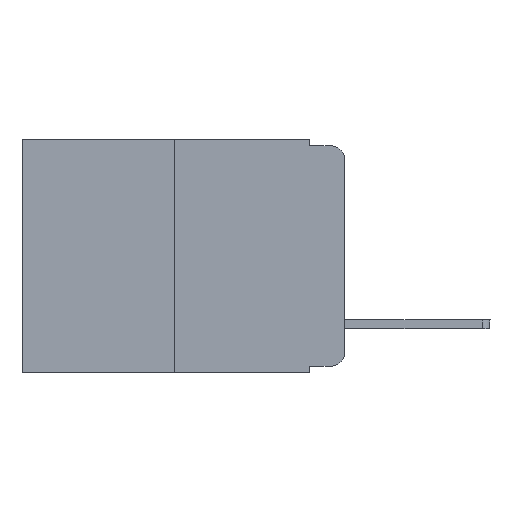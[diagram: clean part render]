
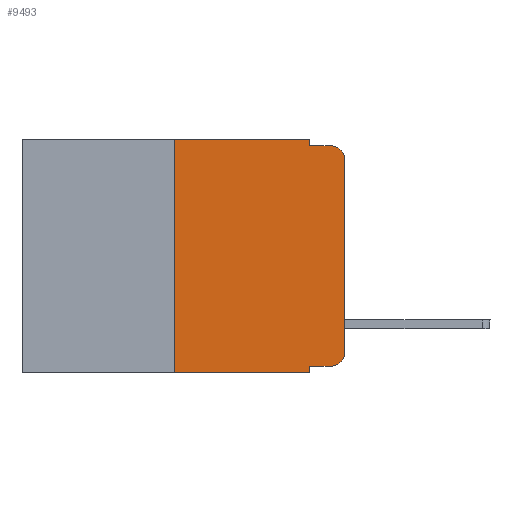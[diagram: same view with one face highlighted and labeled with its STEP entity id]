
A CAD part, left-side view. The second image highlights one B-rep face of the part: STEP entity #9493.
In plain terms, the highlighted planar face has unit normal (-1, 0, 0).
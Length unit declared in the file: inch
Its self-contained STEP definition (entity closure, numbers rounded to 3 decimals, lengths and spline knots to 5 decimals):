
#215 = VECTOR ( 'NONE', #10803, 39.37008 ) ;
#289 = DIRECTION ( 'NONE',  ( 0., 0., 1. ) ) ;
#607 = EDGE_CURVE ( 'NONE', #8277, #5988, #11055, .T. ) ;
#643 = VERTEX_POINT ( 'NONE', #4210 ) ;
#698 = DIRECTION ( 'NONE',  ( 0., 0., -1. ) ) ;
#714 = LINE ( 'NONE', #9930, #3446 ) ;
#875 = DIRECTION ( 'NONE',  ( 1., 0., 0. ) ) ;
#1143 = VECTOR ( 'NONE', #3246, 39.37008 ) ;
#1357 = VERTEX_POINT ( 'NONE', #4005 ) ;
#1798 = ORIENTED_EDGE ( 'NONE', *, *, #607, .F. ) ;
#1890 = EDGE_CURVE ( 'NONE', #4955, #5988, #4414, .T. ) ;
#2115 = AXIS2_PLACEMENT_3D ( 'NONE', #11380, #875, #698 ) ;
#2176 = VECTOR ( 'NONE', #10593, 39.37008 ) ;
#2335 = CARTESIAN_POINT ( 'NONE',  ( 0., 0.051, -0.01 ) ) ;
#2365 = ORIENTED_EDGE ( 'NONE', *, *, #10580, .F. ) ;
#2372 = CARTESIAN_POINT ( 'NONE',  ( 0., 0.25, 0. ) ) ;
#2379 = EDGE_CURVE ( 'NONE', #1357, #10682, #8162, .T. ) ;
#2500 = VERTEX_POINT ( 'NONE', #10598 ) ;
#2794 = LINE ( 'NONE', #2843, #2176 ) ;
#2843 = CARTESIAN_POINT ( 'NONE',  ( 0., 0.473, 0. ) ) ;
#2979 = VERTEX_POINT ( 'NONE', #6728 ) ;
#3246 = DIRECTION ( 'NONE',  ( 0., 0., 1. ) ) ;
#3319 = EDGE_CURVE ( 'NONE', #10682, #2979, #7691, .T. ) ;
#3352 = VECTOR ( 'NONE', #9895, 39.37008 ) ;
#3446 = VECTOR ( 'NONE', #289, 39.37008 ) ;
#3928 = DIRECTION ( 'NONE',  ( 0., -1., 0. ) ) ;
#3960 = CIRCLE ( 'NONE', #7475, 0.02 ) ;
#4005 = CARTESIAN_POINT ( 'NONE',  ( 0., 0.051, 0. ) ) ;
#4210 = CARTESIAN_POINT ( 'NONE',  ( 0., 0.02, -0.333 ) ) ;
#4268 = ORIENTED_EDGE ( 'NONE', *, *, #1890, .T. ) ;
#4309 = DIRECTION ( 'NONE',  ( 0., -1., 0. ) ) ;
#4394 = CARTESIAN_POINT ( 'NONE',  ( 0., 0.02, -0.313 ) ) ;
#4414 = LINE ( 'NONE', #8666, #8028 ) ;
#4492 = DIRECTION ( 'NONE',  ( 0., 0., -1. ) ) ;
#4650 = EDGE_CURVE ( 'NONE', #4955, #5913, #9793, .T. ) ;
#4844 = CARTESIAN_POINT ( 'NONE',  ( 0., 0., -0.03 ) ) ;
#4903 = FACE_OUTER_BOUND ( 'NONE', #11170, .T. ) ;
#4955 = VERTEX_POINT ( 'NONE', #6309 ) ;
#5013 = CARTESIAN_POINT ( 'NONE',  ( 0., 0.051, -0.01 ) ) ;
#5115 = VECTOR ( 'NONE', #4309, 39.37008 ) ;
#5257 = CARTESIAN_POINT ( 'NONE',  ( 0., 0.25, 0. ) ) ;
#5309 = DIRECTION ( 'NONE',  ( -1., 0., 0. ) ) ;
#5337 = LINE ( 'NONE', #6986, #215 ) ;
#5480 = DIRECTION ( 'NONE',  ( 0., 0., -1. ) ) ;
#5795 = ORIENTED_EDGE ( 'NONE', *, *, #2379, .F. ) ;
#5913 = VERTEX_POINT ( 'NONE', #2372 ) ;
#5988 = VERTEX_POINT ( 'NONE', #8321 ) ;
#6107 = CARTESIAN_POINT ( 'NONE',  ( 0., 0.051, 0. ) ) ;
#6309 = CARTESIAN_POINT ( 'NONE',  ( 0., 0.25, -0.343 ) ) ;
#6320 = EDGE_CURVE ( 'NONE', #8277, #643, #5337, .T. ) ;
#6476 = AXIS2_PLACEMENT_3D ( 'NONE', #4394, #5309, #6547 ) ;
#6547 = DIRECTION ( 'NONE',  ( 0., 0., -1. ) ) ;
#6717 = ORIENTED_EDGE ( 'NONE', *, *, #12327, .T. ) ;
#6728 = CARTESIAN_POINT ( 'NONE',  ( 0., 0.02, -0.01 ) ) ;
#6980 = ORIENTED_EDGE ( 'NONE', *, *, #4650, .F. ) ;
#6986 = CARTESIAN_POINT ( 'NONE',  ( 0., 0.051, -0.333 ) ) ;
#7242 = ORIENTED_EDGE ( 'NONE', *, *, #9260, .T. ) ;
#7475 = AXIS2_PLACEMENT_3D ( 'NONE', #10353, #10475, #4492 ) ;
#7691 = LINE ( 'NONE', #2335, #5115 ) ;
#7765 = VERTEX_POINT ( 'NONE', #4844 ) ;
#8028 = VECTOR ( 'NONE', #3928, 39.37008 ) ;
#8162 = LINE ( 'NONE', #11418, #8927 ) ;
#8277 = VERTEX_POINT ( 'NONE', #10317 ) ;
#8321 = CARTESIAN_POINT ( 'NONE',  ( 0., 0.051, -0.343 ) ) ;
#8417 = ORIENTED_EDGE ( 'NONE', *, *, #3319, .F. ) ;
#8626 = EDGE_CURVE ( 'NONE', #2500, #7765, #714, .T. ) ;
#8666 = CARTESIAN_POINT ( 'NONE',  ( 0., 0.473, -0.343 ) ) ;
#8927 = VECTOR ( 'NONE', #5480, 39.37008 ) ;
#9118 = ORIENTED_EDGE ( 'NONE', *, *, #6320, .T. ) ;
#9260 = EDGE_CURVE ( 'NONE', #643, #2500, #10680, .T. ) ;
#9280 = ORIENTED_EDGE ( 'NONE', *, *, #8626, .T. ) ;
#9493 = ADVANCED_FACE ( 'NONE', ( #4903 ), #11420, .F. ) ;
#9793 = LINE ( 'NONE', #5257, #1143 ) ;
#9895 = DIRECTION ( 'NONE',  ( 0., 0., -1. ) ) ;
#9930 = CARTESIAN_POINT ( 'NONE',  ( 0., 0., 0. ) ) ;
#10317 = CARTESIAN_POINT ( 'NONE',  ( 0., 0.051, -0.333 ) ) ;
#10353 = CARTESIAN_POINT ( 'NONE',  ( 0., 0.02, -0.03 ) ) ;
#10475 = DIRECTION ( 'NONE',  ( -1., 0., 0. ) ) ;
#10580 = EDGE_CURVE ( 'NONE', #5913, #1357, #2794, .T. ) ;
#10593 = DIRECTION ( 'NONE',  ( 0., -1., 0. ) ) ;
#10598 = CARTESIAN_POINT ( 'NONE',  ( 0., 0., -0.313 ) ) ;
#10680 = CIRCLE ( 'NONE', #6476, 0.02 ) ;
#10682 = VERTEX_POINT ( 'NONE', #5013 ) ;
#10803 = DIRECTION ( 'NONE',  ( 0., -1., 0. ) ) ;
#11055 = LINE ( 'NONE', #6107, #3352 ) ;
#11170 = EDGE_LOOP ( 'NONE', ( #9280, #6717, #8417, #5795, #2365, #6980, #4268, #1798, #9118, #7242 ) ) ;
#11380 = CARTESIAN_POINT ( 'NONE',  ( 0., 0.473, 0. ) ) ;
#11418 = CARTESIAN_POINT ( 'NONE',  ( 0., 0.051, 0. ) ) ;
#11420 = PLANE ( 'NONE',  #2115 ) ;
#12327 = EDGE_CURVE ( 'NONE', #7765, #2979, #3960, .T. ) ;
